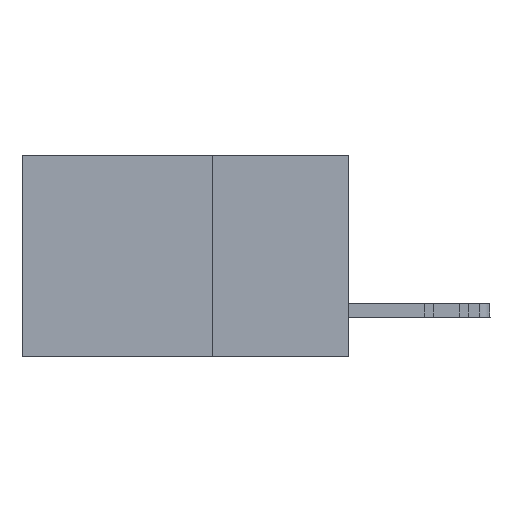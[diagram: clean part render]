
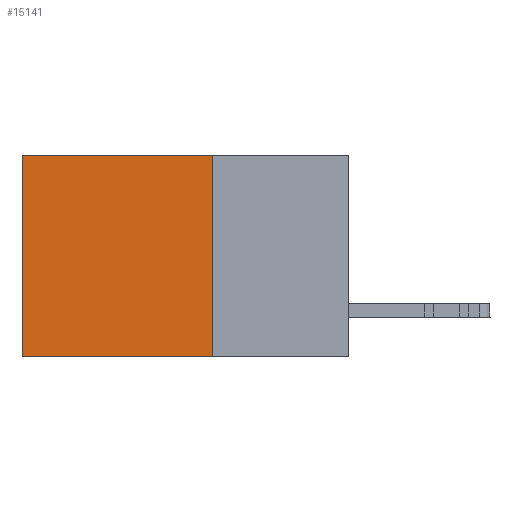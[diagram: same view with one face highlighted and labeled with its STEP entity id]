
A CAD part, left-side view. The second image highlights one B-rep face of the part: STEP entity #15141.
In plain terms, the highlighted planar face has unit normal (-1, 0, 0).
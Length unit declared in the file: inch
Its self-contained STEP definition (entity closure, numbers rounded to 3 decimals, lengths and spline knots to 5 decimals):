
#513 = LINE ( 'NONE', #13445, #17988 ) ;
#856 = EDGE_CURVE ( 'NONE', #25180, #20209, #9982, .T. ) ;
#2704 = DIRECTION ( 'NONE',  ( 1., 0., 0. ) ) ;
#4587 = DIRECTION ( 'NONE',  ( 0., 1., 0. ) ) ;
#4820 = DIRECTION ( 'NONE',  ( 0., 0., -1. ) ) ;
#4945 = CARTESIAN_POINT ( 'NONE',  ( 0.298, 0.6, 0. ) ) ;
#5361 = ORIENTED_EDGE ( 'NONE', *, *, #18392, .T. ) ;
#6196 = VERTEX_POINT ( 'NONE', #9138 ) ;
#6857 = ORIENTED_EDGE ( 'NONE', *, *, #856, .F. ) ;
#9098 = CARTESIAN_POINT ( 'NONE',  ( 0.298, 0.25, 0. ) ) ;
#9138 = CARTESIAN_POINT ( 'NONE',  ( 0.298, 0.6, -0.37 ) ) ;
#9530 = LINE ( 'NONE', #14324, #12287 ) ;
#9982 = LINE ( 'NONE', #23652, #17147 ) ;
#10504 = VERTEX_POINT ( 'NONE', #4945 ) ;
#10929 = LINE ( 'NONE', #13537, #20779 ) ;
#12287 = VECTOR ( 'NONE', #27112, 39.37008 ) ;
#12447 = DIRECTION ( 'NONE',  ( 0., 0., -1. ) ) ;
#13445 = CARTESIAN_POINT ( 'NONE',  ( 0.298, 0.25, 0. ) ) ;
#13537 = CARTESIAN_POINT ( 'NONE',  ( 0.298, 0.6, 0. ) ) ;
#14324 = CARTESIAN_POINT ( 'NONE',  ( 0.298, 0.25, -0.37 ) ) ;
#15141 = ADVANCED_FACE ( 'NONE', ( #19856 ), #20002, .F. ) ;
#15997 = AXIS2_PLACEMENT_3D ( 'NONE', #9098, #2704, #27799 ) ;
#17028 = EDGE_LOOP ( 'NONE', ( #5361, #27845, #6857, #27943 ) ) ;
#17147 = VECTOR ( 'NONE', #12447, 39.37008 ) ;
#17988 = VECTOR ( 'NONE', #4587, 39.37008 ) ;
#18392 = EDGE_CURVE ( 'NONE', #10504, #6196, #10929, .T. ) ;
#19856 = FACE_OUTER_BOUND ( 'NONE', #17028, .T. ) ;
#20002 = PLANE ( 'NONE',  #15997 ) ;
#20209 = VERTEX_POINT ( 'NONE', #25864 ) ;
#20779 = VECTOR ( 'NONE', #4820, 39.37008 ) ;
#20912 = EDGE_CURVE ( 'NONE', #25180, #10504, #513, .T. ) ;
#22408 = CARTESIAN_POINT ( 'NONE',  ( 0.298, 0.25, 0. ) ) ;
#23124 = EDGE_CURVE ( 'NONE', #20209, #6196, #9530, .T. ) ;
#23652 = CARTESIAN_POINT ( 'NONE',  ( 0.298, 0.25, 0. ) ) ;
#25180 = VERTEX_POINT ( 'NONE', #22408 ) ;
#25864 = CARTESIAN_POINT ( 'NONE',  ( 0.298, 0.25, -0.37 ) ) ;
#27112 = DIRECTION ( 'NONE',  ( 0., 1., 0. ) ) ;
#27799 = DIRECTION ( 'NONE',  ( 0., 0., -1. ) ) ;
#27845 = ORIENTED_EDGE ( 'NONE', *, *, #23124, .F. ) ;
#27943 = ORIENTED_EDGE ( 'NONE', *, *, #20912, .T. ) ;
